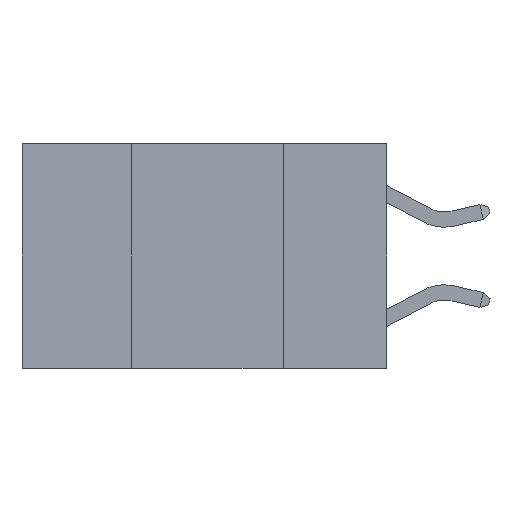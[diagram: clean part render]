
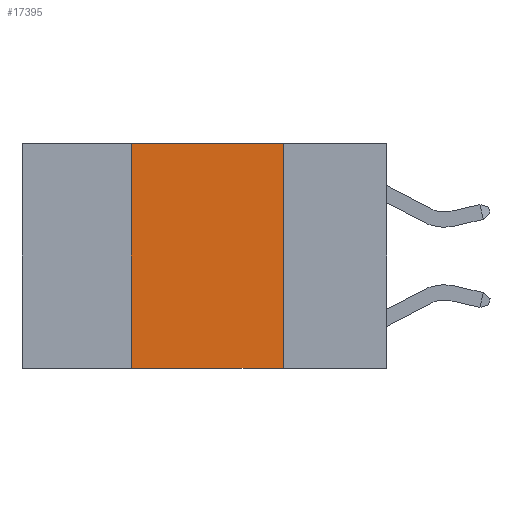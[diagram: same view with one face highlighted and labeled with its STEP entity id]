
A CAD part, left-side view. The second image highlights one B-rep face of the part: STEP entity #17395.
In plain terms, the highlighted planar face has unit normal (-1, 0, 0).
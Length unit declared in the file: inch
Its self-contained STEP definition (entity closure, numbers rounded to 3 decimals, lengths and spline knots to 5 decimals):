
#698 = DIRECTION ( 'NONE',  ( 0., -1., 0. ) ) ;
#1073 = PLANE ( 'NONE',  #23662 ) ;
#1597 = ORIENTED_EDGE ( 'NONE', *, *, #18268, .F. ) ;
#2214 = LINE ( 'NONE', #14665, #13567 ) ;
#2215 = CARTESIAN_POINT ( 'NONE',  ( 0., 0.17, 0. ) ) ;
#2579 = DIRECTION ( 'NONE',  ( 0., 0., -1. ) ) ;
#2603 = CARTESIAN_POINT ( 'NONE',  ( 0., 0.42, -0.37 ) ) ;
#2858 = CARTESIAN_POINT ( 'NONE',  ( 0., 0.17, -0.37 ) ) ;
#3775 = EDGE_LOOP ( 'NONE', ( #20722, #21905, #1597, #20548 ) ) ;
#4952 = DIRECTION ( 'NONE',  ( 0., 0., 1. ) ) ;
#5159 = CARTESIAN_POINT ( 'NONE',  ( 0., 0.6, -0.37 ) ) ;
#6585 = LINE ( 'NONE', #6993, #13326 ) ;
#6930 = DIRECTION ( 'NONE',  ( 0., -1., 0. ) ) ;
#6993 = CARTESIAN_POINT ( 'NONE',  ( 0., 0.42, 0. ) ) ;
#7476 = EDGE_CURVE ( 'NONE', #12161, #7478, #21403, .T. ) ;
#7478 = VERTEX_POINT ( 'NONE', #2858 ) ;
#12161 = VERTEX_POINT ( 'NONE', #2603 ) ;
#12885 = CARTESIAN_POINT ( 'NONE',  ( 0., 0.6, 0. ) ) ;
#13326 = VECTOR ( 'NONE', #4952, 39.37008 ) ;
#13443 = CARTESIAN_POINT ( 'NONE',  ( 0., 0.42, 0. ) ) ;
#13567 = VECTOR ( 'NONE', #698, 39.37008 ) ;
#13622 = EDGE_CURVE ( 'NONE', #17072, #15524, #2214, .T. ) ;
#13661 = VECTOR ( 'NONE', #13666, 39.37008 ) ;
#13666 = DIRECTION ( 'NONE',  ( 0., 0., -1. ) ) ;
#14665 = CARTESIAN_POINT ( 'NONE',  ( 0., 0.6, 0. ) ) ;
#15524 = VERTEX_POINT ( 'NONE', #2215 ) ;
#16290 = EDGE_CURVE ( 'NONE', #15524, #7478, #23969, .T. ) ;
#17072 = VERTEX_POINT ( 'NONE', #13443 ) ;
#17395 = ADVANCED_FACE ( 'NONE', ( #19530 ), #1073, .F. ) ;
#18268 = EDGE_CURVE ( 'NONE', #12161, #17072, #6585, .T. ) ;
#18947 = VECTOR ( 'NONE', #6930, 39.37008 ) ;
#19530 = FACE_OUTER_BOUND ( 'NONE', #3775, .T. ) ;
#20048 = CARTESIAN_POINT ( 'NONE',  ( 0., 0.17, 0. ) ) ;
#20548 = ORIENTED_EDGE ( 'NONE', *, *, #7476, .T. ) ;
#20722 = ORIENTED_EDGE ( 'NONE', *, *, #16290, .F. ) ;
#21403 = LINE ( 'NONE', #5159, #18947 ) ;
#21905 = ORIENTED_EDGE ( 'NONE', *, *, #13622, .F. ) ;
#23662 = AXIS2_PLACEMENT_3D ( 'NONE', #12885, #25891, #2579 ) ;
#23969 = LINE ( 'NONE', #20048, #13661 ) ;
#25891 = DIRECTION ( 'NONE',  ( 1., 0., 0. ) ) ;
